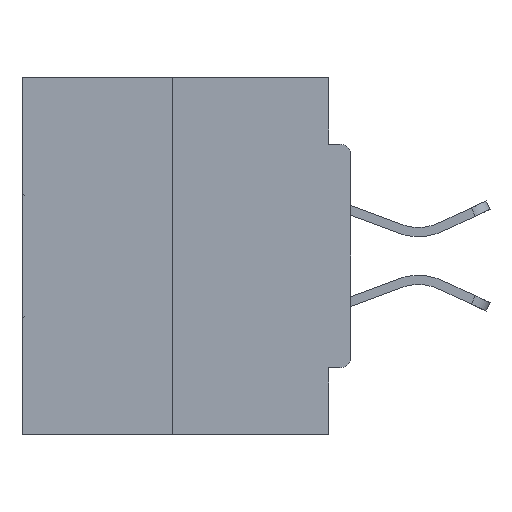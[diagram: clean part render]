
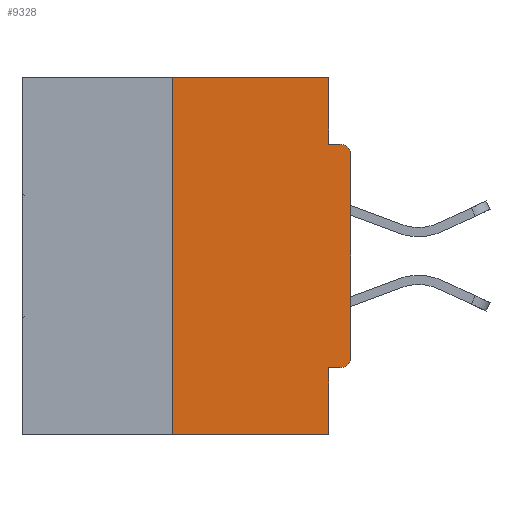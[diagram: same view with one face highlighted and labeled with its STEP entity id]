
A CAD part, left-side view. The second image highlights one B-rep face of the part: STEP entity #9328.
In plain terms, the highlighted planar face has unit normal (-1, 0, 0).
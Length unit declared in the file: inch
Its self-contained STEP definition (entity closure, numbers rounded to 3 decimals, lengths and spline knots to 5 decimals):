
#498 = VERTEX_POINT ( 'NONE', #4612 ) ;
#833 = EDGE_CURVE ( 'NONE', #29199, #14897, #22977, .T. ) ;
#1111 = DIRECTION ( 'NONE',  ( 0., 0., -1. ) ) ;
#1470 = LINE ( 'NONE', #4398, #33405 ) ;
#1578 = LINE ( 'NONE', #1784, #26705 ) ;
#1784 = CARTESIAN_POINT ( 'NONE',  ( 0., 0.031, 0. ) ) ;
#1872 = PLANE ( 'NONE',  #37460 ) ;
#1985 = DIRECTION ( 'NONE',  ( 0., 0., 1. ) ) ;
#3659 = LINE ( 'NONE', #5975, #12937 ) ;
#4193 = ORIENTED_EDGE ( 'NONE', *, *, #10357, .T. ) ;
#4398 = CARTESIAN_POINT ( 'NONE',  ( 0., 0.46, -0.5 ) ) ;
#4612 = CARTESIAN_POINT ( 'NONE',  ( 0., 0.25, 0. ) ) ;
#4814 = CIRCLE ( 'NONE', #34240, 0.015 ) ;
#5837 = CARTESIAN_POINT ( 'NONE',  ( 0., 0.031, 0. ) ) ;
#5975 = CARTESIAN_POINT ( 'NONE',  ( 0., 0., -0.4065 ) ) ;
#6425 = LINE ( 'NONE', #12689, #8610 ) ;
#6489 = EDGE_CURVE ( 'NONE', #9357, #18599, #7021, .T. ) ;
#6555 = EDGE_CURVE ( 'NONE', #36342, #35867, #1578, .T. ) ;
#6979 = EDGE_CURVE ( 'NONE', #498, #36342, #20340, .T. ) ;
#7021 = LINE ( 'NONE', #22701, #9087 ) ;
#7651 = ORIENTED_EDGE ( 'NONE', *, *, #8458, .T. ) ;
#7731 = ORIENTED_EDGE ( 'NONE', *, *, #10153, .F. ) ;
#8257 = VERTEX_POINT ( 'NONE', #40811 ) ;
#8349 = CARTESIAN_POINT ( 'NONE',  ( 0., 0.031, -0.4065 ) ) ;
#8458 = EDGE_CURVE ( 'NONE', #22699, #18599, #1470, .T. ) ;
#8610 = VECTOR ( 'NONE', #9362, 39.37008 ) ;
#9087 = VECTOR ( 'NONE', #31924, 39.37008 ) ;
#9328 = ADVANCED_FACE ( 'NONE', ( #26047 ), #1872, .F. ) ;
#9357 = VERTEX_POINT ( 'NONE', #8349 ) ;
#9362 = DIRECTION ( 'NONE',  ( 0., -1., 0. ) ) ;
#10032 = VECTOR ( 'NONE', #33115, 39.37008 ) ;
#10153 = EDGE_CURVE ( 'NONE', #22699, #498, #21420, .T. ) ;
#10232 = CARTESIAN_POINT ( 'NONE',  ( 0., 0., 0. ) ) ;
#10357 = EDGE_CURVE ( 'NONE', #14897, #8257, #4814, .T. ) ;
#10848 = DIRECTION ( 'NONE',  ( 0., 0., 1. ) ) ;
#11828 = ORIENTED_EDGE ( 'NONE', *, *, #6979, .F. ) ;
#12564 = ORIENTED_EDGE ( 'NONE', *, *, #32495, .F. ) ;
#12689 = CARTESIAN_POINT ( 'NONE',  ( 0., 0., -0.0935 ) ) ;
#12937 = VECTOR ( 'NONE', #22274, 39.37008 ) ;
#14333 = EDGE_LOOP ( 'NONE', ( #11828, #7731, #7651, #34239, #38995, #30279, #14476, #4193, #12564, #31261 ) ) ;
#14476 = ORIENTED_EDGE ( 'NONE', *, *, #833, .T. ) ;
#14897 = VERTEX_POINT ( 'NONE', #27087 ) ;
#15162 = EDGE_CURVE ( 'NONE', #28444, #29199, #32766, .T. ) ;
#16998 = CARTESIAN_POINT ( 'NONE',  ( 0., 0.46, 0. ) ) ;
#17872 = CARTESIAN_POINT ( 'NONE',  ( 0., 0.25, 0. ) ) ;
#17989 = CARTESIAN_POINT ( 'NONE',  ( 0., 0.25, -0.5 ) ) ;
#18599 = VERTEX_POINT ( 'NONE', #32770 ) ;
#19857 = DIRECTION ( 'NONE',  ( 0., -1., 0. ) ) ;
#20340 = LINE ( 'NONE', #16998, #10032 ) ;
#21420 = LINE ( 'NONE', #17872, #30179 ) ;
#22248 = CARTESIAN_POINT ( 'NONE',  ( 0., 0.015, -0.3915 ) ) ;
#22274 = DIRECTION ( 'NONE',  ( 0., 1., 0. ) ) ;
#22699 = VERTEX_POINT ( 'NONE', #17989 ) ;
#22701 = CARTESIAN_POINT ( 'NONE',  ( 0., 0.031, -0.5 ) ) ;
#22977 = LINE ( 'NONE', #10232, #30333 ) ;
#24463 = DIRECTION ( 'NONE',  ( 1., 0., 0. ) ) ;
#24607 = CARTESIAN_POINT ( 'NONE',  ( 0., 0.015, -0.4065 ) ) ;
#25798 = DIRECTION ( 'NONE',  ( -1., 0., 0. ) ) ;
#26047 = FACE_OUTER_BOUND ( 'NONE', #14333, .T. ) ;
#26705 = VECTOR ( 'NONE', #33581, 39.37008 ) ;
#27087 = CARTESIAN_POINT ( 'NONE',  ( 0., 0., -0.1085 ) ) ;
#28444 = VERTEX_POINT ( 'NONE', #24607 ) ;
#28663 = CARTESIAN_POINT ( 'NONE',  ( 0., 0.031, -0.0935 ) ) ;
#29134 = DIRECTION ( 'NONE',  ( -1., 0., 0. ) ) ;
#29199 = VERTEX_POINT ( 'NONE', #30994 ) ;
#30179 = VECTOR ( 'NONE', #1985, 39.37008 ) ;
#30279 = ORIENTED_EDGE ( 'NONE', *, *, #15162, .T. ) ;
#30333 = VECTOR ( 'NONE', #10848, 39.37008 ) ;
#30519 = CARTESIAN_POINT ( 'NONE',  ( 0., 0.46, 0. ) ) ;
#30726 = DIRECTION ( 'NONE',  ( 0., 0., -1. ) ) ;
#30994 = CARTESIAN_POINT ( 'NONE',  ( 0., 0., -0.3915 ) ) ;
#31261 = ORIENTED_EDGE ( 'NONE', *, *, #6555, .F. ) ;
#31924 = DIRECTION ( 'NONE',  ( 0., 0., -1. ) ) ;
#32114 = AXIS2_PLACEMENT_3D ( 'NONE', #22248, #25798, #35002 ) ;
#32289 = CARTESIAN_POINT ( 'NONE',  ( 0., 0.015, -0.1085 ) ) ;
#32495 = EDGE_CURVE ( 'NONE', #35867, #8257, #6425, .T. ) ;
#32766 = CIRCLE ( 'NONE', #32114, 0.015 ) ;
#32770 = CARTESIAN_POINT ( 'NONE',  ( 0., 0.031, -0.5 ) ) ;
#33115 = DIRECTION ( 'NONE',  ( 0., -1., 0. ) ) ;
#33405 = VECTOR ( 'NONE', #19857, 39.37008 ) ;
#33581 = DIRECTION ( 'NONE',  ( 0., 0., -1. ) ) ;
#34239 = ORIENTED_EDGE ( 'NONE', *, *, #6489, .F. ) ;
#34240 = AXIS2_PLACEMENT_3D ( 'NONE', #32289, #29134, #1111 ) ;
#35002 = DIRECTION ( 'NONE',  ( 0., 0., -1. ) ) ;
#35867 = VERTEX_POINT ( 'NONE', #28663 ) ;
#36342 = VERTEX_POINT ( 'NONE', #5837 ) ;
#37460 = AXIS2_PLACEMENT_3D ( 'NONE', #30519, #24463, #30726 ) ;
#38995 = ORIENTED_EDGE ( 'NONE', *, *, #39179, .F. ) ;
#39179 = EDGE_CURVE ( 'NONE', #28444, #9357, #3659, .T. ) ;
#40811 = CARTESIAN_POINT ( 'NONE',  ( 0., 0.015, -0.0935 ) ) ;
